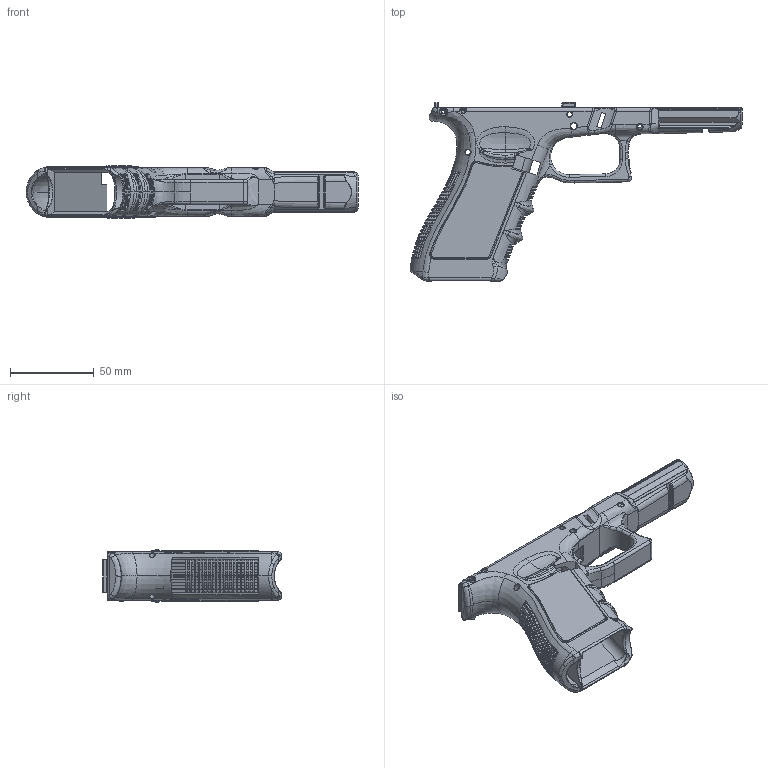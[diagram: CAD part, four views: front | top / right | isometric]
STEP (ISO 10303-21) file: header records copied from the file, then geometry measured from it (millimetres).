
FILE_DESCRIPTION(/* description */ (''),/* implementation_level */ '2;1');
FILE_NAME(/* name */ 'FreeMan''s G17 Frame - button head screws.stp',/* time_stamp */ '2019-03-17T16:23:11-05:00',/* author */ ('johne'),/* organization */ (''),/* preprocessor_version */ 'ST-DEVELOPER v16.13',/* originating_system */ 'Autodesk Inventor 2018',/* authorisation */ '');
FILE_SCHEMA (('AUTOMOTIVE_DESIGN { 1 0 10303 214 3 1 1 }'));
Products named in the file (1): 3D PRINTED 17-RECEIVER SECOND MODEL Rear Mod Buttom Head Bolts v7
Bounding box: 197.79 x 106.5 x 31.4 mm (x, y, z)
Volume: 82396.2 mm3; surface area: 51695.7 mm2
Topology: 1 solids, 1 shells, 2555 faces, 7013 edges, 4432 vertices
Faces by surface type: bspline 1135, plane 845, cylinder 475, torus 42, cone 35, sphere 23
Full cylindrical faces by diameter (mm): 2 x4, 3 x5, 3.2 x2, 3.8 x2
Entity records: 187955 total; most frequent: CARTESIAN_POINT 128959, ORIENTED_EDGE 13882, DIRECTION 10636, EDGE_CURVE 6941, VERTEX_POINT 4414, AXIS2_PLACEMENT_3D 3960, LINE 2716, VECTOR 2716
